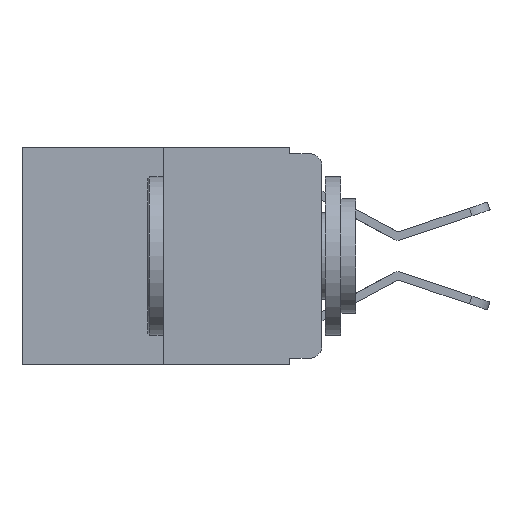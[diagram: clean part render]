
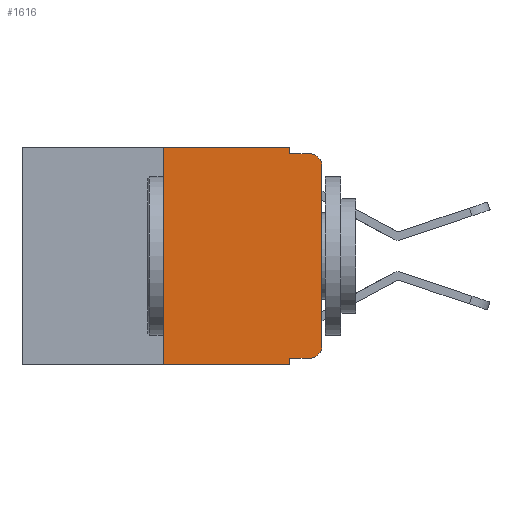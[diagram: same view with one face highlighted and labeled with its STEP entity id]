
A CAD part, left-side view. The second image highlights one B-rep face of the part: STEP entity #1616.
In plain terms, the highlighted planar face has unit normal (-1, 0, 0).
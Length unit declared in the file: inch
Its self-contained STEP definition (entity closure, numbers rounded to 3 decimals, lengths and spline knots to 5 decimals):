
#150 = EDGE_LOOP ( 'NONE', ( #7092, #5727, #11381, #10047, #9364, #9997, #9616, #10553, #2081, #232 ) ) ;
#201 = VERTEX_POINT ( 'NONE', #4397 ) ;
#211 = VERTEX_POINT ( 'NONE', #5593 ) ;
#232 = ORIENTED_EDGE ( 'NONE', *, *, #8454, .T. ) ;
#307 = CARTESIAN_POINT ( 'NONE',  ( 0., 0.051, -0.333 ) ) ;
#463 = VERTEX_POINT ( 'NONE', #2098 ) ;
#482 = DIRECTION ( 'NONE',  ( -1., 0., 0. ) ) ;
#572 = PLANE ( 'NONE',  #6350 ) ;
#877 = EDGE_CURVE ( 'NONE', #6463, #4913, #6949, .T. ) ;
#949 = CARTESIAN_POINT ( 'NONE',  ( 0., 0.473, -0.343 ) ) ;
#964 = LINE ( 'NONE', #2876, #4413 ) ;
#1226 = CARTESIAN_POINT ( 'NONE',  ( 0., 0.25, 0. ) ) ;
#1241 = LINE ( 'NONE', #307, #2627 ) ;
#1363 = EDGE_CURVE ( 'NONE', #9326, #11132, #8292, .T. ) ;
#1449 = CARTESIAN_POINT ( 'NONE',  ( 0., 0.473, 0. ) ) ;
#1616 = ADVANCED_FACE ( 'NONE', ( #3621 ), #572, .F. ) ;
#2081 = ORIENTED_EDGE ( 'NONE', *, *, #8240, .T. ) ;
#2098 = CARTESIAN_POINT ( 'NONE',  ( 0., 0., -0.313 ) ) ;
#2242 = DIRECTION ( 'NONE',  ( 0., -1., 0. ) ) ;
#2364 = LINE ( 'NONE', #949, #3880 ) ;
#2627 = VECTOR ( 'NONE', #3816, 39.37008 ) ;
#2750 = DIRECTION ( 'NONE',  ( 0., 0., -1. ) ) ;
#2834 = EDGE_CURVE ( 'NONE', #211, #8244, #964, .T. ) ;
#2876 = CARTESIAN_POINT ( 'NONE',  ( 0., 0.051, 0. ) ) ;
#3306 = DIRECTION ( 'NONE',  ( 0., 0., -1. ) ) ;
#3342 = DIRECTION ( 'NONE',  ( 1., 0., 0. ) ) ;
#3621 = FACE_OUTER_BOUND ( 'NONE', #150, .T. ) ;
#3659 = VECTOR ( 'NONE', #5837, 39.37008 ) ;
#3816 = DIRECTION ( 'NONE',  ( 0., -1., 0. ) ) ;
#3880 = VECTOR ( 'NONE', #10627, 39.37008 ) ;
#4074 = LINE ( 'NONE', #11282, #3659 ) ;
#4083 = EDGE_CURVE ( 'NONE', #463, #6463, #7538, .T. ) ;
#4190 = CARTESIAN_POINT ( 'NONE',  ( 0., 0.02, -0.01 ) ) ;
#4213 = DIRECTION ( 'NONE',  ( -1., 0., 0. ) ) ;
#4230 = VECTOR ( 'NONE', #2242, 39.37008 ) ;
#4397 = CARTESIAN_POINT ( 'NONE',  ( 0., 0.02, -0.333 ) ) ;
#4413 = VECTOR ( 'NONE', #2750, 39.37008 ) ;
#4913 = VERTEX_POINT ( 'NONE', #4190 ) ;
#5337 = LINE ( 'NONE', #6693, #4230 ) ;
#5433 = DIRECTION ( 'NONE',  ( 0., -1., 0. ) ) ;
#5507 = DIRECTION ( 'NONE',  ( 0., 0., 1. ) ) ;
#5593 = CARTESIAN_POINT ( 'NONE',  ( 0., 0.051, 0. ) ) ;
#5727 = ORIENTED_EDGE ( 'NONE', *, *, #877, .T. ) ;
#5837 = DIRECTION ( 'NONE',  ( 0., 0., -1. ) ) ;
#5991 = DIRECTION ( 'NONE',  ( 0., 0., -1. ) ) ;
#6350 = AXIS2_PLACEMENT_3D ( 'NONE', #1449, #3342, #3306 ) ;
#6463 = VERTEX_POINT ( 'NONE', #10624 ) ;
#6693 = CARTESIAN_POINT ( 'NONE',  ( 0., 0.051, -0.01 ) ) ;
#6695 = EDGE_CURVE ( 'NONE', #7316, #11374, #4074, .T. ) ;
#6949 = CIRCLE ( 'NONE', #7599, 0.02 ) ;
#7092 = ORIENTED_EDGE ( 'NONE', *, *, #4083, .T. ) ;
#7158 = CARTESIAN_POINT ( 'NONE',  ( 0., 0.473, 0. ) ) ;
#7316 = VERTEX_POINT ( 'NONE', #11187 ) ;
#7354 = AXIS2_PLACEMENT_3D ( 'NONE', #9366, #4213, #5991 ) ;
#7538 = LINE ( 'NONE', #7746, #10405 ) ;
#7599 = AXIS2_PLACEMENT_3D ( 'NONE', #8317, #482, #9136 ) ;
#7654 = CARTESIAN_POINT ( 'NONE',  ( 0., 0.051, -0.343 ) ) ;
#7746 = CARTESIAN_POINT ( 'NONE',  ( 0., 0., 0. ) ) ;
#8176 = EDGE_CURVE ( 'NONE', #9326, #11374, #2364, .T. ) ;
#8240 = EDGE_CURVE ( 'NONE', #7316, #201, #1241, .T. ) ;
#8244 = VERTEX_POINT ( 'NONE', #9864 ) ;
#8292 = LINE ( 'NONE', #1226, #9391 ) ;
#8317 = CARTESIAN_POINT ( 'NONE',  ( 0., 0.02, -0.03 ) ) ;
#8454 = EDGE_CURVE ( 'NONE', #201, #463, #9617, .T. ) ;
#8547 = DIRECTION ( 'NONE',  ( 0., 0., 1. ) ) ;
#9012 = LINE ( 'NONE', #7158, #10500 ) ;
#9136 = DIRECTION ( 'NONE',  ( 0., 0., -1. ) ) ;
#9301 = EDGE_CURVE ( 'NONE', #8244, #4913, #5337, .T. ) ;
#9326 = VERTEX_POINT ( 'NONE', #10835 ) ;
#9364 = ORIENTED_EDGE ( 'NONE', *, *, #11139, .F. ) ;
#9366 = CARTESIAN_POINT ( 'NONE',  ( 0., 0.02, -0.313 ) ) ;
#9391 = VECTOR ( 'NONE', #5507, 39.37008 ) ;
#9616 = ORIENTED_EDGE ( 'NONE', *, *, #8176, .T. ) ;
#9617 = CIRCLE ( 'NONE', #7354, 0.02 ) ;
#9864 = CARTESIAN_POINT ( 'NONE',  ( 0., 0.051, -0.01 ) ) ;
#9956 = CARTESIAN_POINT ( 'NONE',  ( 0., 0.25, 0. ) ) ;
#9997 = ORIENTED_EDGE ( 'NONE', *, *, #1363, .F. ) ;
#10047 = ORIENTED_EDGE ( 'NONE', *, *, #2834, .F. ) ;
#10405 = VECTOR ( 'NONE', #8547, 39.37008 ) ;
#10500 = VECTOR ( 'NONE', #5433, 39.37008 ) ;
#10553 = ORIENTED_EDGE ( 'NONE', *, *, #6695, .F. ) ;
#10624 = CARTESIAN_POINT ( 'NONE',  ( 0., 0., -0.03 ) ) ;
#10627 = DIRECTION ( 'NONE',  ( 0., -1., 0. ) ) ;
#10835 = CARTESIAN_POINT ( 'NONE',  ( 0., 0.25, -0.343 ) ) ;
#11132 = VERTEX_POINT ( 'NONE', #9956 ) ;
#11139 = EDGE_CURVE ( 'NONE', #11132, #211, #9012, .T. ) ;
#11187 = CARTESIAN_POINT ( 'NONE',  ( 0., 0.051, -0.333 ) ) ;
#11282 = CARTESIAN_POINT ( 'NONE',  ( 0., 0.051, 0. ) ) ;
#11374 = VERTEX_POINT ( 'NONE', #7654 ) ;
#11381 = ORIENTED_EDGE ( 'NONE', *, *, #9301, .F. ) ;
